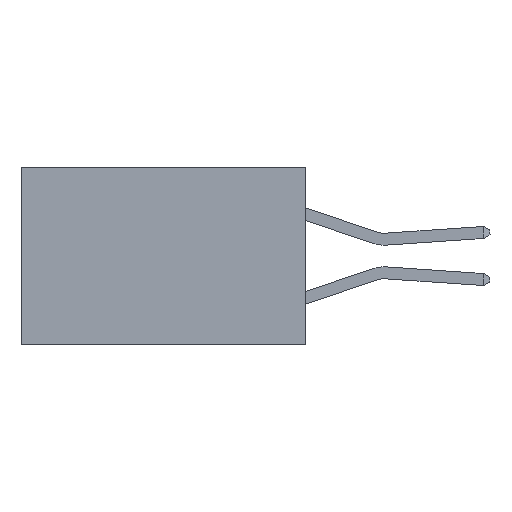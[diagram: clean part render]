
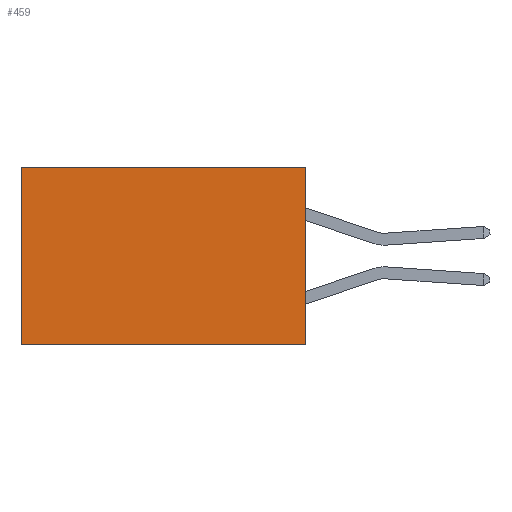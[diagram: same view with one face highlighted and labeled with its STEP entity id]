
A CAD part, left-side view. The second image highlights one B-rep face of the part: STEP entity #459.
In plain terms, the highlighted planar face has unit normal (-1, 0, 0).
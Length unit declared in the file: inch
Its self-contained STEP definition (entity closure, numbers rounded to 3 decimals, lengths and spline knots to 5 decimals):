
#31 = EDGE_CURVE ( 'NONE', #5884, #5384, #3675, .T. ) ;
#319 = DIRECTION ( 'NONE',  ( 0., 1., 0. ) ) ;
#459 = ADVANCED_FACE ( 'NONE', ( #4217 ), #1212, .F. ) ;
#663 = EDGE_CURVE ( 'NONE', #1924, #5247, #1967, .T. ) ;
#1169 = EDGE_CURVE ( 'NONE', #5247, #5384, #5931, .T. ) ;
#1212 = PLANE ( 'NONE',  #8858 ) ;
#1256 = VECTOR ( 'NONE', #319, 39.37008 ) ;
#1358 = ORIENTED_EDGE ( 'NONE', *, *, #1169, .T. ) ;
#1448 = VECTOR ( 'NONE', #4380, 39.37008 ) ;
#1746 = LINE ( 'NONE', #4584, #1448 ) ;
#1924 = VERTEX_POINT ( 'NONE', #2725 ) ;
#1967 = LINE ( 'NONE', #3741, #11343 ) ;
#2502 = ORIENTED_EDGE ( 'NONE', *, *, #4782, .F. ) ;
#2695 = DIRECTION ( 'NONE',  ( 0., 0., -1. ) ) ;
#2725 = CARTESIAN_POINT ( 'NONE',  ( 0.277, 0., 0. ) ) ;
#3642 = ORIENTED_EDGE ( 'NONE', *, *, #663, .T. ) ;
#3675 = LINE ( 'NONE', #8386, #1256 ) ;
#3741 = CARTESIAN_POINT ( 'NONE',  ( 0.277, 0., 0. ) ) ;
#4068 = VECTOR ( 'NONE', #5434, 39.37008 ) ;
#4217 = FACE_OUTER_BOUND ( 'NONE', #8563, .T. ) ;
#4248 = CARTESIAN_POINT ( 'NONE',  ( 0.277, 0., -0.37 ) ) ;
#4380 = DIRECTION ( 'NONE',  ( 0., 0., -1. ) ) ;
#4584 = CARTESIAN_POINT ( 'NONE',  ( 0.277, 0., -0.37 ) ) ;
#4782 = EDGE_CURVE ( 'NONE', #1924, #5884, #1746, .T. ) ;
#4994 = CARTESIAN_POINT ( 'NONE',  ( 0.277, 0.59, -0.37 ) ) ;
#5247 = VERTEX_POINT ( 'NONE', #11008 ) ;
#5384 = VERTEX_POINT ( 'NONE', #10235 ) ;
#5434 = DIRECTION ( 'NONE',  ( 0., 0., -1. ) ) ;
#5884 = VERTEX_POINT ( 'NONE', #7838 ) ;
#5931 = LINE ( 'NONE', #4994, #4068 ) ;
#6534 = ORIENTED_EDGE ( 'NONE', *, *, #31, .F. ) ;
#7485 = DIRECTION ( 'NONE',  ( 0., 1., 0. ) ) ;
#7838 = CARTESIAN_POINT ( 'NONE',  ( 0.277, 0., -0.37 ) ) ;
#7861 = DIRECTION ( 'NONE',  ( 1., 0., 0. ) ) ;
#8386 = CARTESIAN_POINT ( 'NONE',  ( 0.277, 0., -0.37 ) ) ;
#8563 = EDGE_LOOP ( 'NONE', ( #1358, #6534, #2502, #3642 ) ) ;
#8858 = AXIS2_PLACEMENT_3D ( 'NONE', #4248, #7861, #2695 ) ;
#10235 = CARTESIAN_POINT ( 'NONE',  ( 0.277, 0.59, -0.37 ) ) ;
#11008 = CARTESIAN_POINT ( 'NONE',  ( 0.277, 0.59, 0. ) ) ;
#11343 = VECTOR ( 'NONE', #7485, 39.37008 ) ;
